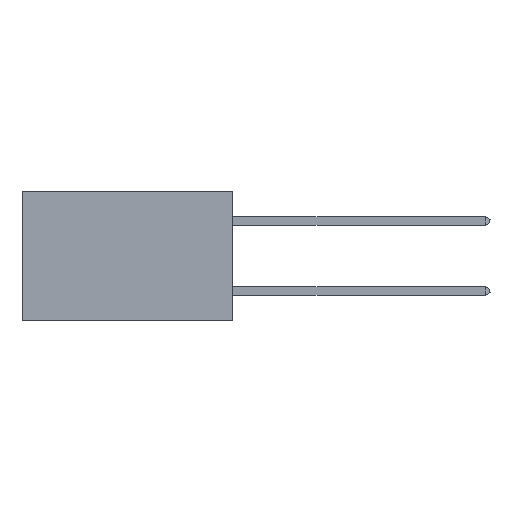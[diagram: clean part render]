
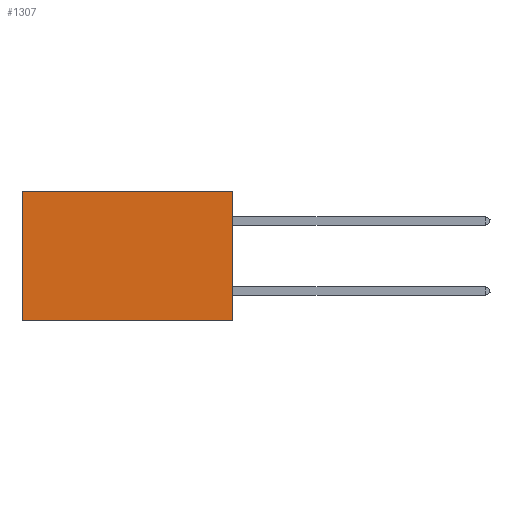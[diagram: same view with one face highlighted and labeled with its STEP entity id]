
A CAD part, left-side view. The second image highlights one B-rep face of the part: STEP entity #1307.
In plain terms, the highlighted planar face has unit normal (-1, 0, 0).
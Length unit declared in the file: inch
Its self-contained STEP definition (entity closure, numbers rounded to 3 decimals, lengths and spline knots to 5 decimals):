
#1307 = ADVANCED_FACE ( 'NONE', ( #9397 ), #21541, .F. ) ;
#1392 = CARTESIAN_POINT ( 'NONE',  ( 0.2875, 0.6, -0.37 ) ) ;
#3521 = EDGE_CURVE ( 'NONE', #19920, #17103, #26445, .T. ) ;
#4588 = VERTEX_POINT ( 'NONE', #38830 ) ;
#6014 = LINE ( 'NONE', #29298, #37360 ) ;
#8613 = AXIS2_PLACEMENT_3D ( 'NONE', #11200, #17616, #21228 ) ;
#8841 = VECTOR ( 'NONE', #9508, 39.37008 ) ;
#9397 = FACE_OUTER_BOUND ( 'NONE', #14979, .T. ) ;
#9508 = DIRECTION ( 'NONE',  ( 0., 1., 0. ) ) ;
#10540 = CARTESIAN_POINT ( 'NONE',  ( 0.2875, 0., 0. ) ) ;
#11200 = CARTESIAN_POINT ( 'NONE',  ( 0.2875, 0., 0. ) ) ;
#13339 = CARTESIAN_POINT ( 'NONE',  ( 0.2875, 0., 0. ) ) ;
#13358 = EDGE_CURVE ( 'NONE', #4588, #22184, #16247, .T. ) ;
#13565 = CARTESIAN_POINT ( 'NONE',  ( 0.2875, 0., -0.37 ) ) ;
#14675 = ORIENTED_EDGE ( 'NONE', *, *, #32193, .F. ) ;
#14979 = EDGE_LOOP ( 'NONE', ( #31456, #14675, #30869, #22219 ) ) ;
#16247 = LINE ( 'NONE', #37436, #39200 ) ;
#16931 = VECTOR ( 'NONE', #46215, 39.37008 ) ;
#17103 = VERTEX_POINT ( 'NONE', #39361 ) ;
#17616 = DIRECTION ( 'NONE',  ( 1., 0., 0. ) ) ;
#19920 = VERTEX_POINT ( 'NONE', #13339 ) ;
#21228 = DIRECTION ( 'NONE',  ( 0., 0., -1. ) ) ;
#21541 = PLANE ( 'NONE',  #8613 ) ;
#22184 = VERTEX_POINT ( 'NONE', #1392 ) ;
#22219 = ORIENTED_EDGE ( 'NONE', *, *, #33240, .T. ) ;
#23180 = DIRECTION ( 'NONE',  ( 0., 0., -1. ) ) ;
#23396 = LINE ( 'NONE', #13565, #8841 ) ;
#26445 = LINE ( 'NONE', #10540, #16931 ) ;
#29298 = CARTESIAN_POINT ( 'NONE',  ( 0.2875, 0., 0. ) ) ;
#30869 = ORIENTED_EDGE ( 'NONE', *, *, #3521, .F. ) ;
#31456 = ORIENTED_EDGE ( 'NONE', *, *, #13358, .T. ) ;
#32193 = EDGE_CURVE ( 'NONE', #17103, #22184, #23396, .T. ) ;
#33240 = EDGE_CURVE ( 'NONE', #19920, #4588, #6014, .T. ) ;
#36514 = DIRECTION ( 'NONE',  ( 0., 1., 0. ) ) ;
#37360 = VECTOR ( 'NONE', #36514, 39.37008 ) ;
#37436 = CARTESIAN_POINT ( 'NONE',  ( 0.2875, 0.6, 0. ) ) ;
#38830 = CARTESIAN_POINT ( 'NONE',  ( 0.2875, 0.6, 0. ) ) ;
#39200 = VECTOR ( 'NONE', #23180, 39.37008 ) ;
#39361 = CARTESIAN_POINT ( 'NONE',  ( 0.2875, 0., -0.37 ) ) ;
#46215 = DIRECTION ( 'NONE',  ( 0., 0., -1. ) ) ;
